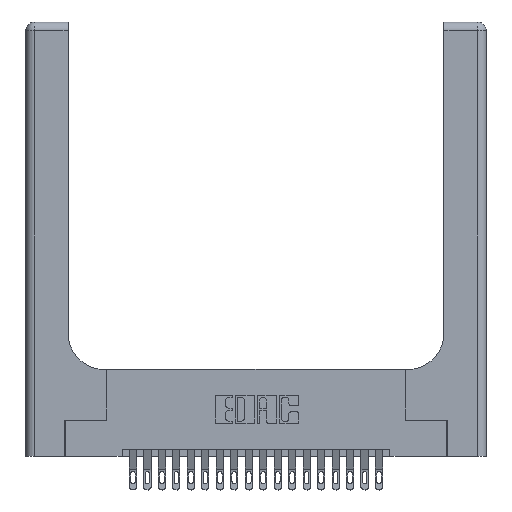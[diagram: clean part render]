
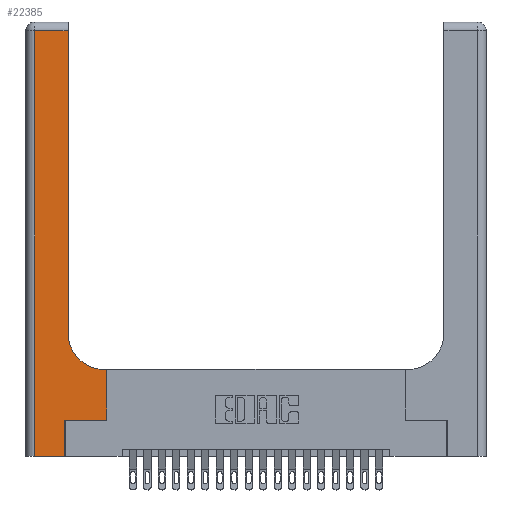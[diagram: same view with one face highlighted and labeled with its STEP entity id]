
A CAD part, top view. The second image highlights one B-rep face of the part: STEP entity #22385.
In plain terms, the highlighted planar face has unit normal (0, 0, 1).
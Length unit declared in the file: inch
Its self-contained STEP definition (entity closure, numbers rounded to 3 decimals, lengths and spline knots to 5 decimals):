
#37 = AXIS2_PLACEMENT_3D ( 'NONE', #9588, #18543, #7969 ) ;
#325 = CIRCLE ( 'NONE', #3752, 0.25 ) ;
#531 = LINE ( 'NONE', #3720, #18904 ) ;
#654 = EDGE_LOOP ( 'NONE', ( #10043, #3931, #6746, #18127, #7910, #5996, #22157, #4026, #6837 ) ) ;
#1275 = VECTOR ( 'NONE', #13774, 39.37008 ) ;
#1478 = EDGE_CURVE ( 'NONE', #21969, #8128, #5216, .T. ) ;
#1793 = EDGE_CURVE ( 'NONE', #6357, #21969, #17401, .T. ) ;
#2329 = EDGE_CURVE ( 'NONE', #12800, #8976, #3207, .T. ) ;
#2601 = VECTOR ( 'NONE', #18675, 39.37008 ) ;
#2802 = CARTESIAN_POINT ( 'NONE',  ( 0., 2.94, 0.37 ) ) ;
#2942 = DIRECTION ( 'NONE',  ( -1., 0., 0. ) ) ;
#3207 = LINE ( 'NONE', #8104, #16840 ) ;
#3229 = VECTOR ( 'NONE', #9975, 39.37008 ) ;
#3463 = DIRECTION ( 'NONE',  ( 0., 0., -1. ) ) ;
#3720 = CARTESIAN_POINT ( 'NONE',  ( 0.06, 3., 0.37 ) ) ;
#3752 = AXIS2_PLACEMENT_3D ( 'NONE', #14139, #3463, #15929 ) ;
#3931 = ORIENTED_EDGE ( 'NONE', *, *, #1478, .T. ) ;
#4026 = ORIENTED_EDGE ( 'NONE', *, *, #5394, .T. ) ;
#5216 = LINE ( 'NONE', #2802, #22768 ) ;
#5394 = EDGE_CURVE ( 'NONE', #8976, #18883, #9810, .T. ) ;
#5729 = CARTESIAN_POINT ( 'NONE',  ( 0.2915, 0.6, 0.37 ) ) ;
#5951 = VERTEX_POINT ( 'NONE', #12477 ) ;
#5996 = ORIENTED_EDGE ( 'NONE', *, *, #11424, .T. ) ;
#6057 = LINE ( 'NONE', #12331, #10186 ) ;
#6357 = VERTEX_POINT ( 'NONE', #10002 ) ;
#6501 = CARTESIAN_POINT ( 'NONE',  ( 0.5415, 0.6, 0.37 ) ) ;
#6746 = ORIENTED_EDGE ( 'NONE', *, *, #15886, .T. ) ;
#6837 = ORIENTED_EDGE ( 'NONE', *, *, #10674, .T. ) ;
#6862 = CARTESIAN_POINT ( 'NONE',  ( 0.06, 2.94, 0.37 ) ) ;
#7669 = CARTESIAN_POINT ( 'NONE',  ( 0.2915, 2.94, 0.37 ) ) ;
#7910 = ORIENTED_EDGE ( 'NONE', *, *, #8014, .T. ) ;
#7969 = DIRECTION ( 'NONE',  ( -1., 0., 0. ) ) ;
#8014 = EDGE_CURVE ( 'NONE', #8114, #16301, #12554, .T. ) ;
#8104 = CARTESIAN_POINT ( 'NONE',  ( 0.5585, 0.25, 0.37 ) ) ;
#8114 = VERTEX_POINT ( 'NONE', #20836 ) ;
#8128 = VERTEX_POINT ( 'NONE', #6862 ) ;
#8489 = CARTESIAN_POINT ( 'NONE',  ( 0.2915, 3., 0.37 ) ) ;
#8560 = DIRECTION ( 'NONE',  ( 0., 1., 0. ) ) ;
#8976 = VERTEX_POINT ( 'NONE', #16440 ) ;
#9244 = VECTOR ( 'NONE', #16342, 39.37008 ) ;
#9588 = CARTESIAN_POINT ( 'NONE',  ( 0., 3., 0.37 ) ) ;
#9810 = LINE ( 'NONE', #5729, #9244 ) ;
#9942 = EDGE_CURVE ( 'NONE', #5951, #8114, #6057, .T. ) ;
#9975 = DIRECTION ( 'NONE',  ( 0., 1., 0. ) ) ;
#10002 = CARTESIAN_POINT ( 'NONE',  ( 0.2915, 0.85, 0.37 ) ) ;
#10043 = ORIENTED_EDGE ( 'NONE', *, *, #1793, .T. ) ;
#10186 = VECTOR ( 'NONE', #14097, 39.37008 ) ;
#10674 = EDGE_CURVE ( 'NONE', #18883, #6357, #325, .T. ) ;
#10693 = CARTESIAN_POINT ( 'NONE',  ( 0.5585, 0.25, 0.37 ) ) ;
#11424 = EDGE_CURVE ( 'NONE', #16301, #12800, #16786, .T. ) ;
#11835 = FACE_OUTER_BOUND ( 'NONE', #654, .T. ) ;
#11983 = CARTESIAN_POINT ( 'NONE',  ( 0.269, 0., 0.37 ) ) ;
#12331 = CARTESIAN_POINT ( 'NONE',  ( 0., 0., 0.37 ) ) ;
#12477 = CARTESIAN_POINT ( 'NONE',  ( 0.06, 0., 0.37 ) ) ;
#12554 = LINE ( 'NONE', #11983, #1275 ) ;
#12800 = VERTEX_POINT ( 'NONE', #10693 ) ;
#13774 = DIRECTION ( 'NONE',  ( 0., 1., 0. ) ) ;
#14097 = DIRECTION ( 'NONE',  ( 1., 0., 0. ) ) ;
#14139 = CARTESIAN_POINT ( 'NONE',  ( 0.5415, 0.85, 0.37 ) ) ;
#15886 = EDGE_CURVE ( 'NONE', #8128, #5951, #531, .T. ) ;
#15929 = DIRECTION ( 'NONE',  ( 1., 0., 0. ) ) ;
#16301 = VERTEX_POINT ( 'NONE', #19302 ) ;
#16342 = DIRECTION ( 'NONE',  ( -1., 0., 0. ) ) ;
#16440 = CARTESIAN_POINT ( 'NONE',  ( 0.5585, 0.6, 0.37 ) ) ;
#16786 = LINE ( 'NONE', #16932, #2601 ) ;
#16804 = PLANE ( 'NONE',  #37 ) ;
#16840 = VECTOR ( 'NONE', #8560, 39.37008 ) ;
#16932 = CARTESIAN_POINT ( 'NONE',  ( 0.269, 0.25, 0.37 ) ) ;
#17401 = LINE ( 'NONE', #8489, #3229 ) ;
#18127 = ORIENTED_EDGE ( 'NONE', *, *, #9942, .T. ) ;
#18543 = DIRECTION ( 'NONE',  ( 0., 0., -1. ) ) ;
#18675 = DIRECTION ( 'NONE',  ( 1., 0., 0. ) ) ;
#18883 = VERTEX_POINT ( 'NONE', #6501 ) ;
#18904 = VECTOR ( 'NONE', #21337, 39.37008 ) ;
#19302 = CARTESIAN_POINT ( 'NONE',  ( 0.269, 0.25, 0.37 ) ) ;
#20836 = CARTESIAN_POINT ( 'NONE',  ( 0.269, 0., 0.37 ) ) ;
#21337 = DIRECTION ( 'NONE',  ( 0., -1., 0. ) ) ;
#21969 = VERTEX_POINT ( 'NONE', #7669 ) ;
#22157 = ORIENTED_EDGE ( 'NONE', *, *, #2329, .T. ) ;
#22385 = ADVANCED_FACE ( 'NONE', ( #11835 ), #16804, .F. ) ;
#22768 = VECTOR ( 'NONE', #2942, 39.37008 ) ;
